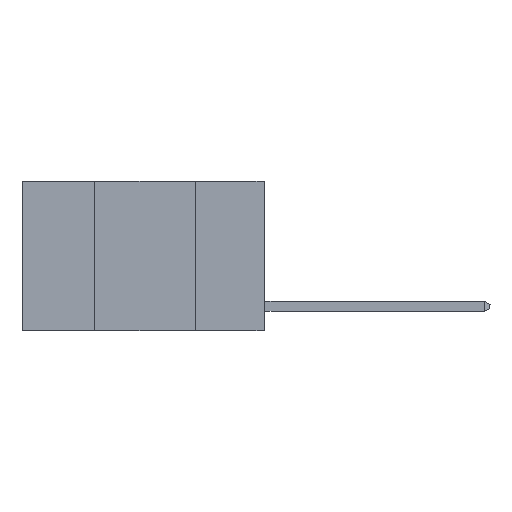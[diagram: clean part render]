
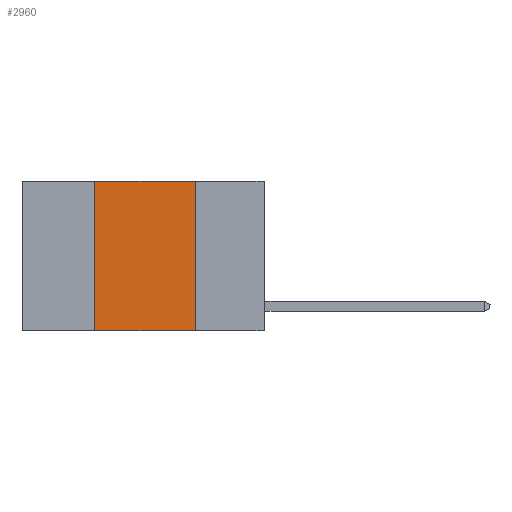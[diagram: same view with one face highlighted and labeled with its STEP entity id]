
A CAD part, left-side view. The second image highlights one B-rep face of the part: STEP entity #2960.
In plain terms, the highlighted planar face has unit normal (-1, 0, 0).
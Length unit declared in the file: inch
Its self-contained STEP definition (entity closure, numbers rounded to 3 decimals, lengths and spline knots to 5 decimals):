
#158 = VERTEX_POINT ( 'NONE', #10782 ) ;
#689 = CARTESIAN_POINT ( 'NONE',  ( 0., 0.17, 0. ) ) ;
#711 = CARTESIAN_POINT ( 'NONE',  ( 0., 0.6, 0. ) ) ;
#1322 = EDGE_CURVE ( 'NONE', #5614, #3407, #1477, .T. ) ;
#1477 = LINE ( 'NONE', #7513, #6084 ) ;
#1838 = CARTESIAN_POINT ( 'NONE',  ( 0., 0.42, -0.37 ) ) ;
#1874 = EDGE_CURVE ( 'NONE', #9008, #3407, #7321, .T. ) ;
#2213 = EDGE_LOOP ( 'NONE', ( #5439, #5457, #7641, #4977 ) ) ;
#2960 = ADVANCED_FACE ( 'NONE', ( #3000 ), #10362, .F. ) ;
#3000 = FACE_OUTER_BOUND ( 'NONE', #2213, .T. ) ;
#3240 = LINE ( 'NONE', #711, #5735 ) ;
#3407 = VERTEX_POINT ( 'NONE', #3977 ) ;
#3745 = DIRECTION ( 'NONE',  ( 0., 0., 1. ) ) ;
#3943 = EDGE_CURVE ( 'NONE', #158, #5614, #3240, .T. ) ;
#3977 = CARTESIAN_POINT ( 'NONE',  ( 0., 0.17, -0.37 ) ) ;
#4288 = VECTOR ( 'NONE', #6528, 39.37008 ) ;
#4977 = ORIENTED_EDGE ( 'NONE', *, *, #1874, .T. ) ;
#5154 = EDGE_CURVE ( 'NONE', #9008, #158, #8489, .T. ) ;
#5439 = ORIENTED_EDGE ( 'NONE', *, *, #1322, .F. ) ;
#5457 = ORIENTED_EDGE ( 'NONE', *, *, #3943, .F. ) ;
#5614 = VERTEX_POINT ( 'NONE', #689 ) ;
#5735 = VECTOR ( 'NONE', #8971, 39.37008 ) ;
#6084 = VECTOR ( 'NONE', #9219, 39.37008 ) ;
#6528 = DIRECTION ( 'NONE',  ( 0., -1., 0. ) ) ;
#7254 = CARTESIAN_POINT ( 'NONE',  ( 0., 0.6, -0.37 ) ) ;
#7321 = LINE ( 'NONE', #7254, #4288 ) ;
#7513 = CARTESIAN_POINT ( 'NONE',  ( 0., 0.17, 0. ) ) ;
#7641 = ORIENTED_EDGE ( 'NONE', *, *, #5154, .F. ) ;
#7858 = DIRECTION ( 'NONE',  ( 0., 0., -1. ) ) ;
#8217 = VECTOR ( 'NONE', #3745, 39.37008 ) ;
#8489 = LINE ( 'NONE', #10275, #8217 ) ;
#8671 = CARTESIAN_POINT ( 'NONE',  ( 0., 0.6, 0. ) ) ;
#8971 = DIRECTION ( 'NONE',  ( 0., -1., 0. ) ) ;
#9008 = VERTEX_POINT ( 'NONE', #1838 ) ;
#9219 = DIRECTION ( 'NONE',  ( 0., 0., -1. ) ) ;
#10275 = CARTESIAN_POINT ( 'NONE',  ( 0., 0.42, 0. ) ) ;
#10362 = PLANE ( 'NONE',  #10880 ) ;
#10393 = DIRECTION ( 'NONE',  ( 1., 0., 0. ) ) ;
#10782 = CARTESIAN_POINT ( 'NONE',  ( 0., 0.42, 0. ) ) ;
#10880 = AXIS2_PLACEMENT_3D ( 'NONE', #8671, #10393, #7858 ) ;
